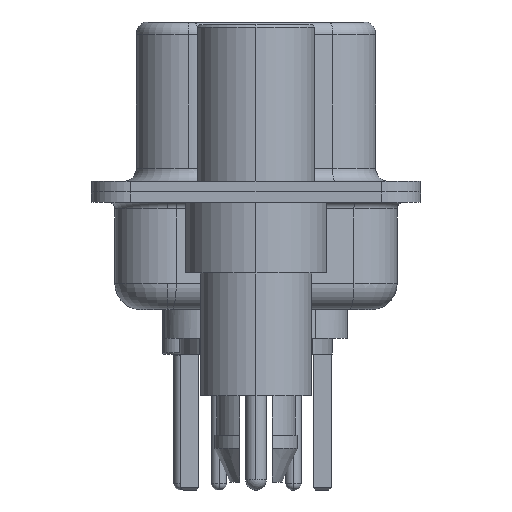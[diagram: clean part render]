
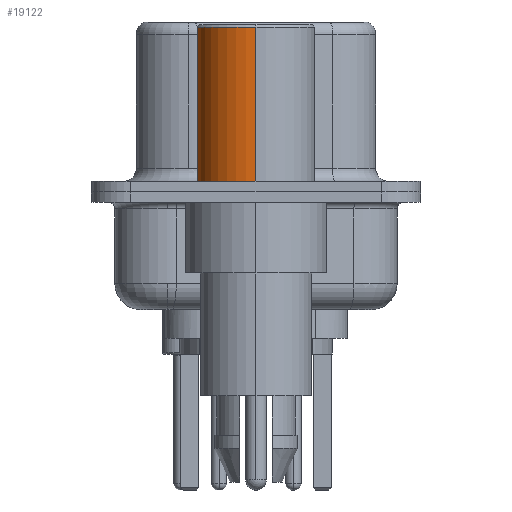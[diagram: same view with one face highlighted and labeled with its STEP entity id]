
A CAD part, left-side view. The second image highlights one B-rep face of the part: STEP entity #19122.
In plain terms, the highlighted cylindrical face has radius 2.25 mm (diameter 4.5 mm), a partial arc.
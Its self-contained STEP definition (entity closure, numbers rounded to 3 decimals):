
#626 = AXIS2_PLACEMENT_3D ( 'NONE', #9216, #7405, #14751 ) ;
#2599 = EDGE_LOOP ( 'NONE', ( #12352, #7422, #19572, #10949 ) ) ;
#3020 = LINE ( 'NONE', #15745, #3327 ) ;
#3327 = VECTOR ( 'NONE', #13716, 1000. ) ;
#3698 = EDGE_CURVE ( 'NONE', #13155, #9463, #4993, .T. ) ;
#4476 = CARTESIAN_POINT ( 'NONE',  ( -2.25, 0., 0.4 ) ) ;
#4993 = CIRCLE ( 'NONE', #14400, 2.25 ) ;
#5689 = CARTESIAN_POINT ( 'NONE',  ( 2.25, 0., 0.581 ) ) ;
#7358 = CARTESIAN_POINT ( 'NONE',  ( -2.25, 0., 6.3 ) ) ;
#7405 = DIRECTION ( 'NONE',  ( 0., 0., 1. ) ) ;
#7422 = ORIENTED_EDGE ( 'NONE', *, *, #12183, .T. ) ;
#7909 = EDGE_CURVE ( 'NONE', #15491, #13155, #19506, .T. ) ;
#7944 = EDGE_CURVE ( 'NONE', #15491, #19594, #12365, .T. ) ;
#8982 = CARTESIAN_POINT ( 'NONE',  ( 2.25, 0., 0.4 ) ) ;
#9216 = CARTESIAN_POINT ( 'NONE',  ( 0., 0., 0.581 ) ) ;
#9463 = VERTEX_POINT ( 'NONE', #7358 ) ;
#10949 = ORIENTED_EDGE ( 'NONE', *, *, #7909, .F. ) ;
#11790 = CYLINDRICAL_SURFACE ( 'NONE', #626, 2.25 ) ;
#12120 = CARTESIAN_POINT ( 'NONE',  ( 0., 0., 6.3 ) ) ;
#12183 = EDGE_CURVE ( 'NONE', #19594, #9463, #3020, .T. ) ;
#12352 = ORIENTED_EDGE ( 'NONE', *, *, #7944, .T. ) ;
#12365 = CIRCLE ( 'NONE', #18659, 2.25 ) ;
#13155 = VERTEX_POINT ( 'NONE', #18679 ) ;
#13716 = DIRECTION ( 'NONE',  ( 0., 0., 1. ) ) ;
#14400 = AXIS2_PLACEMENT_3D ( 'NONE', #12120, #15902, #14801 ) ;
#14751 = DIRECTION ( 'NONE',  ( 1., 0., 0. ) ) ;
#14801 = DIRECTION ( 'NONE',  ( 1., 0., 0. ) ) ;
#15353 = DIRECTION ( 'NONE',  ( 1., 0., 0. ) ) ;
#15491 = VERTEX_POINT ( 'NONE', #8982 ) ;
#15745 = CARTESIAN_POINT ( 'NONE',  ( -2.25, 0., 0.581 ) ) ;
#15902 = DIRECTION ( 'NONE',  ( 0., 0., 1. ) ) ;
#17134 = DIRECTION ( 'NONE',  ( 0., 0., 1. ) ) ;
#18099 = FACE_OUTER_BOUND ( 'NONE', #2599, .T. ) ;
#18659 = AXIS2_PLACEMENT_3D ( 'NONE', #22590, #17134, #15353 ) ;
#18679 = CARTESIAN_POINT ( 'NONE',  ( 2.25, 0., 6.3 ) ) ;
#19122 = ADVANCED_FACE ( 'NONE', ( #18099 ), #11790, .T. ) ;
#19506 = LINE ( 'NONE', #5689, #20337 ) ;
#19572 = ORIENTED_EDGE ( 'NONE', *, *, #3698, .F. ) ;
#19594 = VERTEX_POINT ( 'NONE', #4476 ) ;
#20298 = DIRECTION ( 'NONE',  ( 0., 0., 1. ) ) ;
#20337 = VECTOR ( 'NONE', #20298, 1000. ) ;
#22590 = CARTESIAN_POINT ( 'NONE',  ( 0., 0., 0.4 ) ) ;
